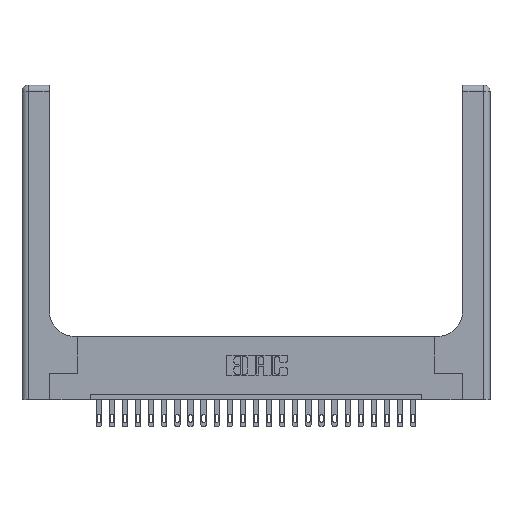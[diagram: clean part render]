
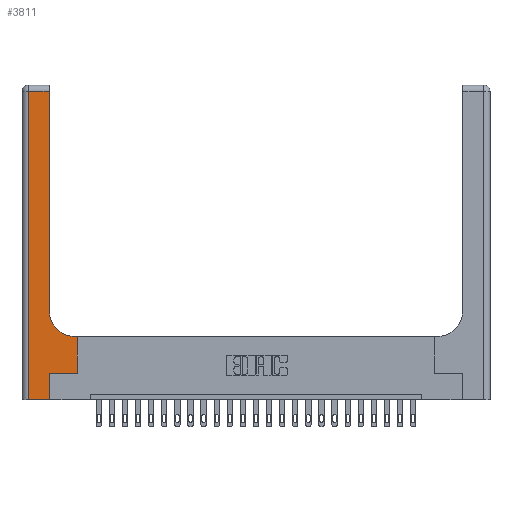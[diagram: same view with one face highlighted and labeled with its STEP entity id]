
A CAD part, top view. The second image highlights one B-rep face of the part: STEP entity #3811.
In plain terms, the highlighted planar face has unit normal (0, 0, 1).
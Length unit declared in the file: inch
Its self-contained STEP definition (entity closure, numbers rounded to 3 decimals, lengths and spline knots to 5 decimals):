
#99 = ORIENTED_EDGE ( 'NONE', *, *, #19414, .T. ) ;
#593 = CARTESIAN_POINT ( 'NONE',  ( 0.06, 2.94, 0.37 ) ) ;
#690 = VECTOR ( 'NONE', #19375, 39.37008 ) ;
#775 = FACE_OUTER_BOUND ( 'NONE', #8677, .T. ) ;
#833 = CARTESIAN_POINT ( 'NONE',  ( 0.06, 3., 0.37 ) ) ;
#894 = CARTESIAN_POINT ( 'NONE',  ( 0., 3., 0.37 ) ) ;
#1005 = LINE ( 'NONE', #9756, #8565 ) ;
#1748 = CIRCLE ( 'NONE', #7394, 0.25 ) ;
#1985 = LINE ( 'NONE', #14522, #8124 ) ;
#2100 = ORIENTED_EDGE ( 'NONE', *, *, #11146, .T. ) ;
#2318 = AXIS2_PLACEMENT_3D ( 'NONE', #894, #18819, #15205 ) ;
#2587 = ORIENTED_EDGE ( 'NONE', *, *, #6220, .T. ) ;
#3811 = ADVANCED_FACE ( 'NONE', ( #775 ), #13547, .F. ) ;
#4071 = ORIENTED_EDGE ( 'NONE', *, *, #22562, .T. ) ;
#4348 = VERTEX_POINT ( 'NONE', #20603 ) ;
#4367 = CARTESIAN_POINT ( 'NONE',  ( 0.26, 2.94, 0.37 ) ) ;
#4734 = CARTESIAN_POINT ( 'NONE',  ( 0.528, 0.6, 0.37 ) ) ;
#5128 = DIRECTION ( 'NONE',  ( 1., 0., 0. ) ) ;
#5513 = CARTESIAN_POINT ( 'NONE',  ( 0., 0., 0.37 ) ) ;
#5781 = DIRECTION ( 'NONE',  ( -1., 0., 0. ) ) ;
#6220 = EDGE_CURVE ( 'NONE', #10702, #9821, #18036, .T. ) ;
#6449 = CARTESIAN_POINT ( 'NONE',  ( 0.51, 0.85, 0.37 ) ) ;
#6961 = VECTOR ( 'NONE', #21206, 39.37008 ) ;
#7310 = CARTESIAN_POINT ( 'NONE',  ( 0.51, 0.6, 0.37 ) ) ;
#7394 = AXIS2_PLACEMENT_3D ( 'NONE', #6449, #19421, #5128 ) ;
#7414 = VECTOR ( 'NONE', #15207, 39.37008 ) ;
#7553 = DIRECTION ( 'NONE',  ( -1., 0., 0. ) ) ;
#7703 = ORIENTED_EDGE ( 'NONE', *, *, #15425, .T. ) ;
#8124 = VECTOR ( 'NONE', #7553, 39.37008 ) ;
#8453 = LINE ( 'NONE', #14097, #6961 ) ;
#8565 = VECTOR ( 'NONE', #20980, 39.37008 ) ;
#8677 = EDGE_LOOP ( 'NONE', ( #4071, #21221, #17273, #2587, #17553, #7703, #2100, #99, #22642 ) ) ;
#8805 = EDGE_CURVE ( 'NONE', #10290, #10702, #15142, .T. ) ;
#8817 = CARTESIAN_POINT ( 'NONE',  ( 0.265, 0.25, 0.37 ) ) ;
#9164 = VERTEX_POINT ( 'NONE', #7310 ) ;
#9640 = LINE ( 'NONE', #18696, #7414 ) ;
#9756 = CARTESIAN_POINT ( 'NONE',  ( 0.528, 0.25, 0.37 ) ) ;
#9821 = VERTEX_POINT ( 'NONE', #21077 ) ;
#10257 = EDGE_CURVE ( 'NONE', #22760, #10290, #11462, .T. ) ;
#10290 = VERTEX_POINT ( 'NONE', #593 ) ;
#10702 = VERTEX_POINT ( 'NONE', #21133 ) ;
#10949 = VECTOR ( 'NONE', #16379, 39.37008 ) ;
#11146 = EDGE_CURVE ( 'NONE', #4348, #13119, #1005, .T. ) ;
#11462 = LINE ( 'NONE', #20331, #19062 ) ;
#11466 = DIRECTION ( 'NONE',  ( 0., -1., 0. ) ) ;
#11673 = VERTEX_POINT ( 'NONE', #15507 ) ;
#12185 = CARTESIAN_POINT ( 'NONE',  ( 0.26, 3., 0.37 ) ) ;
#12555 = VERTEX_POINT ( 'NONE', #8817 ) ;
#13119 = VERTEX_POINT ( 'NONE', #4734 ) ;
#13547 = PLANE ( 'NONE',  #2318 ) ;
#14097 = CARTESIAN_POINT ( 'NONE',  ( 0.265, 0., 0.37 ) ) ;
#14429 = EDGE_CURVE ( 'NONE', #9164, #11673, #1748, .T. ) ;
#14522 = CARTESIAN_POINT ( 'NONE',  ( 0.26, 0.6, 0.37 ) ) ;
#15142 = LINE ( 'NONE', #833, #20086 ) ;
#15205 = DIRECTION ( 'NONE',  ( -1., 0., 0. ) ) ;
#15207 = DIRECTION ( 'NONE',  ( 1., 0., 0. ) ) ;
#15425 = EDGE_CURVE ( 'NONE', #12555, #4348, #9640, .T. ) ;
#15507 = CARTESIAN_POINT ( 'NONE',  ( 0.26, 0.85, 0.37 ) ) ;
#16379 = DIRECTION ( 'NONE',  ( 1., 0., 0. ) ) ;
#17273 = ORIENTED_EDGE ( 'NONE', *, *, #8805, .T. ) ;
#17553 = ORIENTED_EDGE ( 'NONE', *, *, #18833, .T. ) ;
#18036 = LINE ( 'NONE', #5513, #10949 ) ;
#18696 = CARTESIAN_POINT ( 'NONE',  ( 0.265, 0.25, 0.37 ) ) ;
#18819 = DIRECTION ( 'NONE',  ( 0., 0., -1. ) ) ;
#18833 = EDGE_CURVE ( 'NONE', #9821, #12555, #8453, .T. ) ;
#19062 = VECTOR ( 'NONE', #5781, 39.37008 ) ;
#19375 = DIRECTION ( 'NONE',  ( 0., 1., 0. ) ) ;
#19414 = EDGE_CURVE ( 'NONE', #13119, #9164, #1985, .T. ) ;
#19421 = DIRECTION ( 'NONE',  ( 0., 0., -1. ) ) ;
#19488 = LINE ( 'NONE', #12185, #690 ) ;
#20086 = VECTOR ( 'NONE', #11466, 39.37008 ) ;
#20331 = CARTESIAN_POINT ( 'NONE',  ( 0., 2.94, 0.37 ) ) ;
#20603 = CARTESIAN_POINT ( 'NONE',  ( 0.528, 0.25, 0.37 ) ) ;
#20980 = DIRECTION ( 'NONE',  ( 0., 1., 0. ) ) ;
#21077 = CARTESIAN_POINT ( 'NONE',  ( 0.265, 0., 0.37 ) ) ;
#21133 = CARTESIAN_POINT ( 'NONE',  ( 0.06, 0., 0.37 ) ) ;
#21206 = DIRECTION ( 'NONE',  ( 0., 1., 0. ) ) ;
#21221 = ORIENTED_EDGE ( 'NONE', *, *, #10257, .T. ) ;
#22562 = EDGE_CURVE ( 'NONE', #11673, #22760, #19488, .T. ) ;
#22642 = ORIENTED_EDGE ( 'NONE', *, *, #14429, .T. ) ;
#22760 = VERTEX_POINT ( 'NONE', #4367 ) ;
